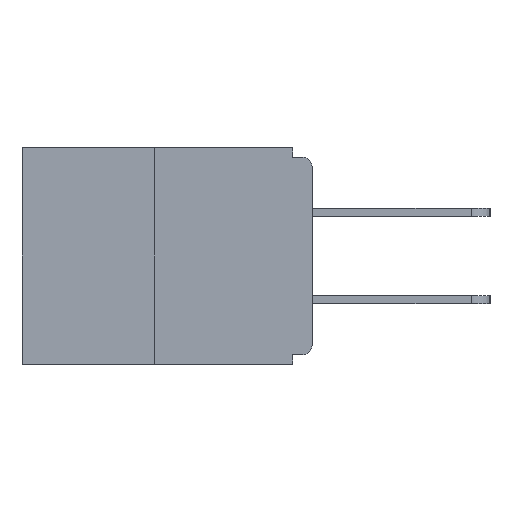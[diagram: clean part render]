
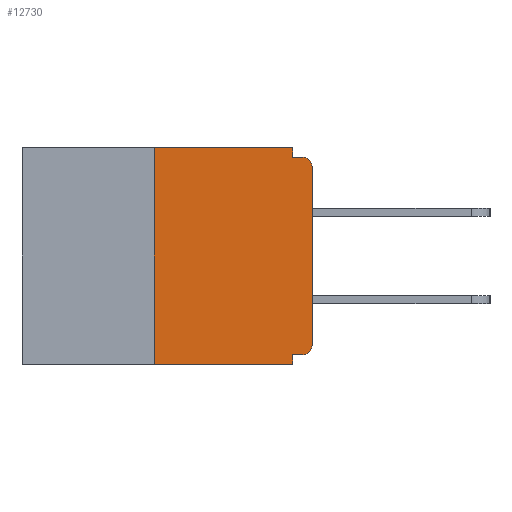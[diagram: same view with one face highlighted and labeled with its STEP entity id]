
A CAD part, left-side view. The second image highlights one B-rep face of the part: STEP entity #12730.
In plain terms, the highlighted planar face has unit normal (-1, 0, 0).
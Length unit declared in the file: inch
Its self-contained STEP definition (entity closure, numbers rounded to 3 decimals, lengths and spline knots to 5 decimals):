
#132 = EDGE_CURVE ( 'NONE', #2502, #1991, #11640, .T. ) ;
#340 = EDGE_LOOP ( 'NONE', ( #4660, #2617, #2812, #2871, #8376, #8954, #9111, #7417, #12774, #8953 ) ) ;
#449 = EDGE_CURVE ( 'NONE', #2574, #5457, #11943, .T. ) ;
#699 = DIRECTION ( 'NONE',  ( -1., 0., 0. ) ) ;
#718 = VERTEX_POINT ( 'NONE', #6254 ) ;
#788 = DIRECTION ( 'NONE',  ( -1., 0., 0. ) ) ;
#954 = CARTESIAN_POINT ( 'NONE',  ( 0., 0.031, -0.343 ) ) ;
#971 = DIRECTION ( 'NONE',  ( 0., 0., 1. ) ) ;
#1049 = CARTESIAN_POINT ( 'NONE',  ( 0., 0., -0.328 ) ) ;
#1114 = LINE ( 'NONE', #2879, #12440 ) ;
#1160 = LINE ( 'NONE', #1049, #4012 ) ;
#1239 = VECTOR ( 'NONE', #8772, 39.37008 ) ;
#1256 = EDGE_CURVE ( 'NONE', #2238, #718, #11463, .T. ) ;
#1298 = VERTEX_POINT ( 'NONE', #9799 ) ;
#1602 = CARTESIAN_POINT ( 'NONE',  ( 0., 0.031, -0.328 ) ) ;
#1737 = DIRECTION ( 'NONE',  ( 0., 0., -1. ) ) ;
#1890 = CIRCLE ( 'NONE', #3602, 0.015 ) ;
#1901 = PLANE ( 'NONE',  #8437 ) ;
#1934 = EDGE_CURVE ( 'NONE', #2574, #8050, #10661, .T. ) ;
#1991 = VERTEX_POINT ( 'NONE', #7203 ) ;
#2238 = VERTEX_POINT ( 'NONE', #7538 ) ;
#2502 = VERTEX_POINT ( 'NONE', #3138 ) ;
#2574 = VERTEX_POINT ( 'NONE', #3444 ) ;
#2617 = ORIENTED_EDGE ( 'NONE', *, *, #1934, .F. ) ;
#2766 = CARTESIAN_POINT ( 'NONE',  ( 0., 0.015, -0.015 ) ) ;
#2812 = ORIENTED_EDGE ( 'NONE', *, *, #449, .T. ) ;
#2871 = ORIENTED_EDGE ( 'NONE', *, *, #12648, .F. ) ;
#2879 = CARTESIAN_POINT ( 'NONE',  ( 0., 0., 0. ) ) ;
#2937 = DIRECTION ( 'NONE',  ( 0., 0., 1. ) ) ;
#3138 = CARTESIAN_POINT ( 'NONE',  ( 0., 0.031, 0. ) ) ;
#3444 = CARTESIAN_POINT ( 'NONE',  ( 0., 0.25, -0.343 ) ) ;
#3463 = EDGE_CURVE ( 'NONE', #718, #1298, #1114, .T. ) ;
#3557 = CARTESIAN_POINT ( 'NONE',  ( 0., 0.031, -0.343 ) ) ;
#3602 = AXIS2_PLACEMENT_3D ( 'NONE', #12654, #788, #12614 ) ;
#3873 = DIRECTION ( 'NONE',  ( 1., 0., 0. ) ) ;
#3909 = VECTOR ( 'NONE', #10464, 39.37008 ) ;
#4012 = VECTOR ( 'NONE', #7962, 39.37008 ) ;
#4080 = DIRECTION ( 'NONE',  ( 0., -1., 0. ) ) ;
#4204 = EDGE_CURVE ( 'NONE', #1298, #10497, #1890, .T. ) ;
#4558 = DIRECTION ( 'NONE',  ( 0., 0., -1. ) ) ;
#4660 = ORIENTED_EDGE ( 'NONE', *, *, #5680, .F. ) ;
#5363 = AXIS2_PLACEMENT_3D ( 'NONE', #8543, #699, #5581 ) ;
#5457 = VERTEX_POINT ( 'NONE', #954 ) ;
#5581 = DIRECTION ( 'NONE',  ( 0., 0., -1. ) ) ;
#5680 = EDGE_CURVE ( 'NONE', #8050, #2502, #7449, .T. ) ;
#5865 = VECTOR ( 'NONE', #2937, 39.37008 ) ;
#6121 = CARTESIAN_POINT ( 'NONE',  ( 0., 0., -0.015 ) ) ;
#6211 = FACE_OUTER_BOUND ( 'NONE', #340, .T. ) ;
#6254 = CARTESIAN_POINT ( 'NONE',  ( 0., 0., -0.313 ) ) ;
#6496 = VECTOR ( 'NONE', #4080, 39.37008 ) ;
#6741 = CARTESIAN_POINT ( 'NONE',  ( 0., 0.25, 0. ) ) ;
#6777 = EDGE_CURVE ( 'NONE', #1991, #10497, #10198, .T. ) ;
#7203 = CARTESIAN_POINT ( 'NONE',  ( 0., 0.031, -0.015 ) ) ;
#7357 = CARTESIAN_POINT ( 'NONE',  ( 0., 0.031, 0. ) ) ;
#7417 = ORIENTED_EDGE ( 'NONE', *, *, #4204, .T. ) ;
#7449 = LINE ( 'NONE', #11998, #10538 ) ;
#7538 = CARTESIAN_POINT ( 'NONE',  ( 0., 0.015, -0.328 ) ) ;
#7934 = EDGE_CURVE ( 'NONE', #2238, #11288, #1160, .T. ) ;
#7962 = DIRECTION ( 'NONE',  ( 0., 1., 0. ) ) ;
#8050 = VERTEX_POINT ( 'NONE', #12059 ) ;
#8376 = ORIENTED_EDGE ( 'NONE', *, *, #7934, .F. ) ;
#8437 = AXIS2_PLACEMENT_3D ( 'NONE', #8841, #3873, #1737 ) ;
#8543 = CARTESIAN_POINT ( 'NONE',  ( 0., 0.015, -0.313 ) ) ;
#8772 = DIRECTION ( 'NONE',  ( 0., -1., 0. ) ) ;
#8841 = CARTESIAN_POINT ( 'NONE',  ( 0., 0.46, 0. ) ) ;
#8953 = ORIENTED_EDGE ( 'NONE', *, *, #132, .F. ) ;
#8954 = ORIENTED_EDGE ( 'NONE', *, *, #1256, .T. ) ;
#9111 = ORIENTED_EDGE ( 'NONE', *, *, #3463, .T. ) ;
#9174 = LINE ( 'NONE', #3557, #3909 ) ;
#9183 = DIRECTION ( 'NONE',  ( 0., -1., 0. ) ) ;
#9799 = CARTESIAN_POINT ( 'NONE',  ( 0., 0., -0.03 ) ) ;
#9902 = CARTESIAN_POINT ( 'NONE',  ( 0., 0.46, -0.343 ) ) ;
#10198 = LINE ( 'NONE', #6121, #6496 ) ;
#10464 = DIRECTION ( 'NONE',  ( 0., 0., -1. ) ) ;
#10497 = VERTEX_POINT ( 'NONE', #2766 ) ;
#10538 = VECTOR ( 'NONE', #9183, 39.37008 ) ;
#10661 = LINE ( 'NONE', #6741, #5865 ) ;
#11288 = VERTEX_POINT ( 'NONE', #1602 ) ;
#11463 = CIRCLE ( 'NONE', #5363, 0.015 ) ;
#11640 = LINE ( 'NONE', #7357, #12256 ) ;
#11943 = LINE ( 'NONE', #9902, #1239 ) ;
#11998 = CARTESIAN_POINT ( 'NONE',  ( 0., 0.46, 0. ) ) ;
#12059 = CARTESIAN_POINT ( 'NONE',  ( 0., 0.25, 0. ) ) ;
#12256 = VECTOR ( 'NONE', #4558, 39.37008 ) ;
#12440 = VECTOR ( 'NONE', #971, 39.37008 ) ;
#12614 = DIRECTION ( 'NONE',  ( 0., 0., -1. ) ) ;
#12648 = EDGE_CURVE ( 'NONE', #11288, #5457, #9174, .T. ) ;
#12654 = CARTESIAN_POINT ( 'NONE',  ( 0., 0.015, -0.03 ) ) ;
#12730 = ADVANCED_FACE ( 'NONE', ( #6211 ), #1901, .F. ) ;
#12774 = ORIENTED_EDGE ( 'NONE', *, *, #6777, .F. ) ;
